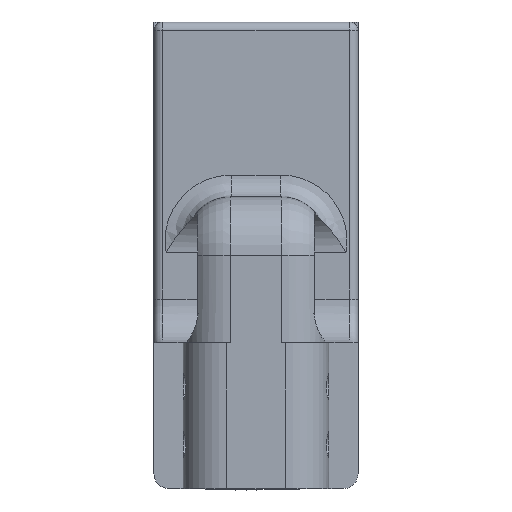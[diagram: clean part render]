
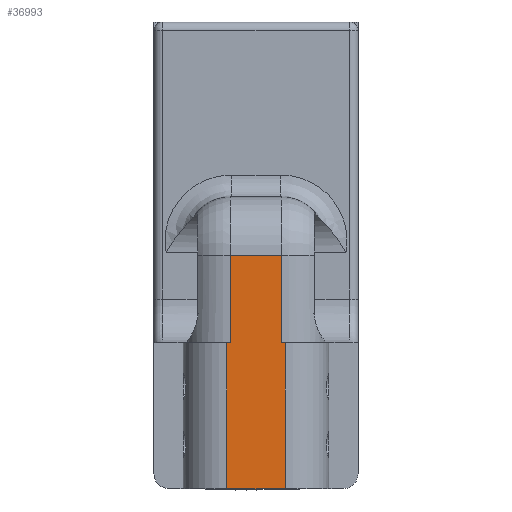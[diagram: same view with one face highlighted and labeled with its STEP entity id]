
A CAD part, front view. The second image highlights one B-rep face of the part: STEP entity #36993.
In plain terms, the highlighted planar face has unit normal (0, -1, 0).
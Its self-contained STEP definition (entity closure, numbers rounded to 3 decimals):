
#262 = CARTESIAN_POINT ( 'NONE',  ( 45., -58.378, -90.097 ) ) ;
#364 = CARTESIAN_POINT ( 'NONE',  ( 43.82, -58.378, -10.097 ) ) ;
#817 = VECTOR ( 'NONE', #18858, 1000. ) ;
#1067 = CARTESIAN_POINT ( 'NONE',  ( 25., -58.378, -90.097 ) ) ;
#1859 = ORIENTED_EDGE ( 'NONE', *, *, #13285, .T. ) ;
#2358 = FACE_OUTER_BOUND ( 'NONE', #9427, .T. ) ;
#2433 = LINE ( 'NONE', #34255, #19134 ) ;
#2633 = DIRECTION ( 'NONE',  ( -1., 0., 0. ) ) ;
#3388 = EDGE_CURVE ( 'NONE', #31290, #11753, #12799, .T. ) ;
#3493 = EDGE_CURVE ( 'NONE', #11753, #27411, #37526, .T. ) ;
#3770 = EDGE_CURVE ( 'NONE', #27411, #9376, #37038, .T. ) ;
#4452 = EDGE_CURVE ( 'NONE', #9376, #30229, #12759, .T. ) ;
#4500 = VERTEX_POINT ( 'NONE', #34927 ) ;
#4731 = DIRECTION ( 'NONE',  ( 1., 0., 0. ) ) ;
#4833 = VECTOR ( 'NONE', #28425, 1000. ) ;
#4876 = VECTOR ( 'NONE', #4731, 1000. ) ;
#6125 = VECTOR ( 'NONE', #18714, 1000. ) ;
#8276 = PLANE ( 'NONE',  #8626 ) ;
#8405 = DIRECTION ( 'NONE',  ( 0., 1., 0. ) ) ;
#8626 = AXIS2_PLACEMENT_3D ( 'NONE', #26264, #8405, #29289 ) ;
#8694 = LINE ( 'NONE', #21867, #817 ) ;
#9360 = VECTOR ( 'NONE', #2633, 1000. ) ;
#9376 = VERTEX_POINT ( 'NONE', #12602 ) ;
#9427 = EDGE_LOOP ( 'NONE', ( #14062, #1859, #33766, #13167, #16067, #22274, #21595, #12123 ) ) ;
#10456 = CARTESIAN_POINT ( 'NONE',  ( 45., -58.378, -40.097 ) ) ;
#11216 = CARTESIAN_POINT ( 'NONE',  ( 45., -58.378, -40.097 ) ) ;
#11753 = VERTEX_POINT ( 'NONE', #262 ) ;
#12123 = ORIENTED_EDGE ( 'NONE', *, *, #4452, .T. ) ;
#12602 = CARTESIAN_POINT ( 'NONE',  ( 43.82, -58.378, -40.097 ) ) ;
#12759 = LINE ( 'NONE', #25671, #4833 ) ;
#12799 = LINE ( 'NONE', #22317, #4876 ) ;
#13107 = LINE ( 'NONE', #1067, #6125 ) ;
#13167 = ORIENTED_EDGE ( 'NONE', *, *, #34682, .T. ) ;
#13285 = EDGE_CURVE ( 'NONE', #4500, #24391, #8694, .T. ) ;
#14062 = ORIENTED_EDGE ( 'NONE', *, *, #20579, .T. ) ;
#16067 = ORIENTED_EDGE ( 'NONE', *, *, #3388, .T. ) ;
#16349 = DIRECTION ( 'NONE',  ( -1., 0., 0. ) ) ;
#18216 = CARTESIAN_POINT ( 'NONE',  ( 25., -58.378, -40.097 ) ) ;
#18714 = DIRECTION ( 'NONE',  ( 0., 0., -1. ) ) ;
#18827 = VECTOR ( 'NONE', #29108, 1000. ) ;
#18858 = DIRECTION ( 'NONE',  ( 0., 0., -1. ) ) ;
#19134 = VECTOR ( 'NONE', #16349, 1000. ) ;
#19569 = DIRECTION ( 'NONE',  ( -1., 0., 0. ) ) ;
#20401 = CARTESIAN_POINT ( 'NONE',  ( 0., -58.378, -10.097 ) ) ;
#20579 = EDGE_CURVE ( 'NONE', #30229, #4500, #32243, .T. ) ;
#21166 = VECTOR ( 'NONE', #19569, 1000. ) ;
#21595 = ORIENTED_EDGE ( 'NONE', *, *, #3770, .T. ) ;
#21792 = VERTEX_POINT ( 'NONE', #18216 ) ;
#21867 = CARTESIAN_POINT ( 'NONE',  ( 26.18, -58.378, 0. ) ) ;
#22274 = ORIENTED_EDGE ( 'NONE', *, *, #3493, .T. ) ;
#22317 = CARTESIAN_POINT ( 'NONE',  ( 0., -58.378, -90.097 ) ) ;
#24391 = VERTEX_POINT ( 'NONE', #34099 ) ;
#25671 = CARTESIAN_POINT ( 'NONE',  ( 43.82, -58.378, 0. ) ) ;
#26264 = CARTESIAN_POINT ( 'NONE',  ( 0., -58.378, 0. ) ) ;
#27411 = VERTEX_POINT ( 'NONE', #10456 ) ;
#28425 = DIRECTION ( 'NONE',  ( 0., 0., 1. ) ) ;
#29108 = DIRECTION ( 'NONE',  ( 0., 0., 1. ) ) ;
#29289 = DIRECTION ( 'NONE',  ( 0., 0., 1. ) ) ;
#30229 = VERTEX_POINT ( 'NONE', #364 ) ;
#30595 = CARTESIAN_POINT ( 'NONE',  ( 0., -58.378, -40.097 ) ) ;
#31290 = VERTEX_POINT ( 'NONE', #33943 ) ;
#32243 = LINE ( 'NONE', #20401, #9360 ) ;
#33766 = ORIENTED_EDGE ( 'NONE', *, *, #34810, .T. ) ;
#33943 = CARTESIAN_POINT ( 'NONE',  ( 25., -58.378, -90.097 ) ) ;
#34099 = CARTESIAN_POINT ( 'NONE',  ( 26.18, -58.378, -40.097 ) ) ;
#34255 = CARTESIAN_POINT ( 'NONE',  ( 0., -58.378, -40.097 ) ) ;
#34682 = EDGE_CURVE ( 'NONE', #21792, #31290, #13107, .T. ) ;
#34810 = EDGE_CURVE ( 'NONE', #24391, #21792, #2433, .T. ) ;
#34927 = CARTESIAN_POINT ( 'NONE',  ( 26.18, -58.378, -10.097 ) ) ;
#36993 = ADVANCED_FACE ( 'NONE', ( #2358 ), #8276, .F. ) ;
#37038 = LINE ( 'NONE', #30595, #21166 ) ;
#37526 = LINE ( 'NONE', #11216, #18827 ) ;
